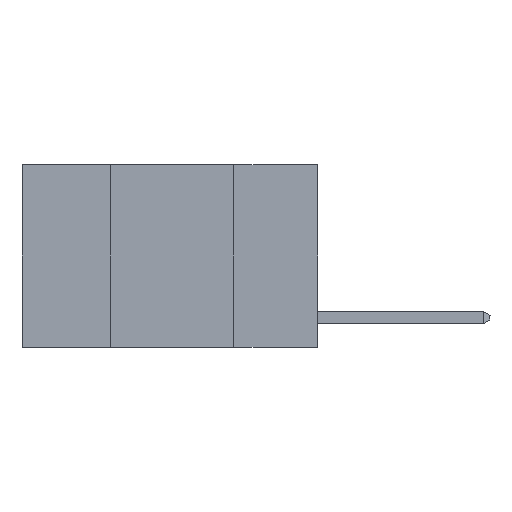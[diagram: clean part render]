
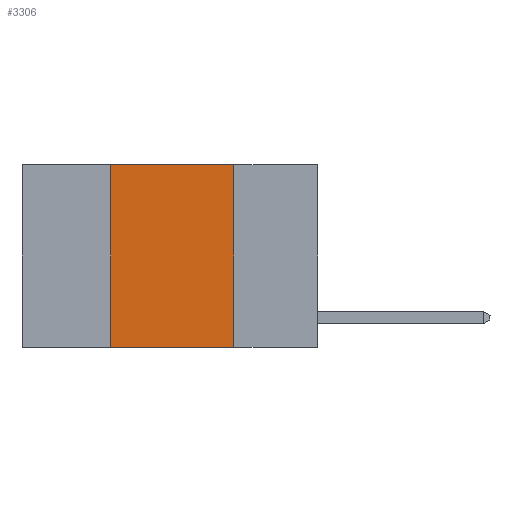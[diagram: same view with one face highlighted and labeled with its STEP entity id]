
A CAD part, left-side view. The second image highlights one B-rep face of the part: STEP entity #3306.
In plain terms, the highlighted planar face has unit normal (-1, 0, 0).
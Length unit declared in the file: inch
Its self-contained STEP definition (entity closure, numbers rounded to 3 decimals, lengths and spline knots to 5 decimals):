
#1380 = PLANE ( 'NONE',  #7934 ) ;
#1539 = LINE ( 'NONE', #20356, #7716 ) ;
#2204 = VERTEX_POINT ( 'NONE', #19497 ) ;
#2589 = VECTOR ( 'NONE', #18338, 39.37008 ) ;
#3306 = ADVANCED_FACE ( 'NONE', ( #18592 ), #1380, .F. ) ;
#4582 = DIRECTION ( 'NONE',  ( 0., 0., 1. ) ) ;
#5019 = DIRECTION ( 'NONE',  ( 0., 0., -1. ) ) ;
#6707 = VECTOR ( 'NONE', #20467, 39.37008 ) ;
#7716 = VECTOR ( 'NONE', #18255, 39.37008 ) ;
#7764 = CARTESIAN_POINT ( 'NONE',  ( 0., 0.42, -0.37 ) ) ;
#7934 = AXIS2_PLACEMENT_3D ( 'NONE', #14973, #16717, #5019 ) ;
#8585 = ORIENTED_EDGE ( 'NONE', *, *, #8914, .T. ) ;
#8688 = VERTEX_POINT ( 'NONE', #7764 ) ;
#8914 = EDGE_CURVE ( 'NONE', #8688, #10946, #1539, .T. ) ;
#10799 = EDGE_CURVE ( 'NONE', #2204, #10946, #14593, .T. ) ;
#10946 = VERTEX_POINT ( 'NONE', #16499 ) ;
#11078 = CARTESIAN_POINT ( 'NONE',  ( 0., 0.6, 0. ) ) ;
#12574 = VERTEX_POINT ( 'NONE', #14732 ) ;
#13342 = ORIENTED_EDGE ( 'NONE', *, *, #19698, .F. ) ;
#13866 = EDGE_CURVE ( 'NONE', #12574, #2204, #14870, .T. ) ;
#14463 = CARTESIAN_POINT ( 'NONE',  ( 0., 0.17, 0. ) ) ;
#14593 = LINE ( 'NONE', #14463, #2589 ) ;
#14732 = CARTESIAN_POINT ( 'NONE',  ( 0., 0.42, 0. ) ) ;
#14870 = LINE ( 'NONE', #11078, #6707 ) ;
#14973 = CARTESIAN_POINT ( 'NONE',  ( 0., 0.6, 0. ) ) ;
#15687 = VECTOR ( 'NONE', #4582, 39.37008 ) ;
#16499 = CARTESIAN_POINT ( 'NONE',  ( 0., 0.17, -0.37 ) ) ;
#16717 = DIRECTION ( 'NONE',  ( 1., 0., 0. ) ) ;
#17502 = ORIENTED_EDGE ( 'NONE', *, *, #13866, .F. ) ;
#17657 = LINE ( 'NONE', #18026, #15687 ) ;
#17666 = ORIENTED_EDGE ( 'NONE', *, *, #10799, .F. ) ;
#18026 = CARTESIAN_POINT ( 'NONE',  ( 0., 0.42, 0. ) ) ;
#18255 = DIRECTION ( 'NONE',  ( 0., -1., 0. ) ) ;
#18338 = DIRECTION ( 'NONE',  ( 0., 0., -1. ) ) ;
#18592 = FACE_OUTER_BOUND ( 'NONE', #21462, .T. ) ;
#19497 = CARTESIAN_POINT ( 'NONE',  ( 0., 0.17, 0. ) ) ;
#19698 = EDGE_CURVE ( 'NONE', #8688, #12574, #17657, .T. ) ;
#20356 = CARTESIAN_POINT ( 'NONE',  ( 0., 0.6, -0.37 ) ) ;
#20467 = DIRECTION ( 'NONE',  ( 0., -1., 0. ) ) ;
#21462 = EDGE_LOOP ( 'NONE', ( #17666, #17502, #13342, #8585 ) ) ;
